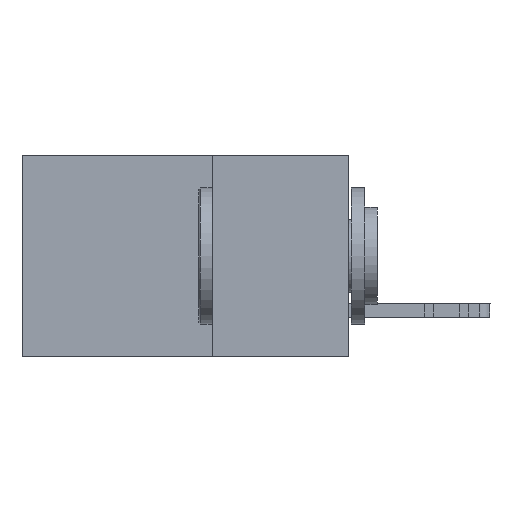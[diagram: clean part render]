
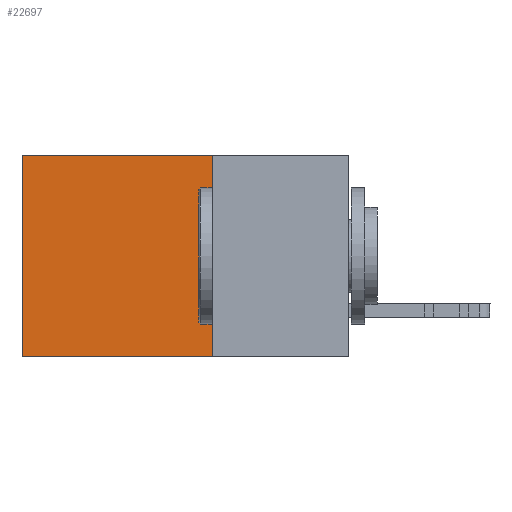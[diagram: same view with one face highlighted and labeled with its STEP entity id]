
A CAD part, left-side view. The second image highlights one B-rep face of the part: STEP entity #22697.
In plain terms, the highlighted planar face has unit normal (-1, 0, 0).
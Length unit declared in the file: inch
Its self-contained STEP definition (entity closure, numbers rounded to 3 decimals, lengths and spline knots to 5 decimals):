
#252 = VERTEX_POINT ( 'NONE', #21242 ) ;
#1880 = ORIENTED_EDGE ( 'NONE', *, *, #21041, .F. ) ;
#3267 = CARTESIAN_POINT ( 'NONE',  ( 0.2615, 0.25, -0.37 ) ) ;
#6181 = LINE ( 'NONE', #14293, #18385 ) ;
#7783 = VERTEX_POINT ( 'NONE', #18566 ) ;
#7862 = DIRECTION ( 'NONE',  ( 0., 0., -1. ) ) ;
#8875 = VERTEX_POINT ( 'NONE', #10356 ) ;
#9104 = AXIS2_PLACEMENT_3D ( 'NONE', #13878, #12019, #26201 ) ;
#9757 = FACE_OUTER_BOUND ( 'NONE', #20924, .T. ) ;
#10244 = ORIENTED_EDGE ( 'NONE', *, *, #13152, .T. ) ;
#10356 = CARTESIAN_POINT ( 'NONE',  ( 0.2615, 0.6, -0.37 ) ) ;
#11650 = DIRECTION ( 'NONE',  ( 0., 1., 0. ) ) ;
#12019 = DIRECTION ( 'NONE',  ( 1., 0., 0. ) ) ;
#12041 = VECTOR ( 'NONE', #7862, 39.37008 ) ;
#12356 = CARTESIAN_POINT ( 'NONE',  ( 0.2615, 0.25, -0.37 ) ) ;
#12427 = VECTOR ( 'NONE', #11650, 39.37008 ) ;
#13152 = EDGE_CURVE ( 'NONE', #7783, #8875, #13577, .T. ) ;
#13577 = LINE ( 'NONE', #25514, #12041 ) ;
#13782 = DIRECTION ( 'NONE',  ( 0., 1., 0. ) ) ;
#13878 = CARTESIAN_POINT ( 'NONE',  ( 0.2615, 0.25, -0.37 ) ) ;
#14007 = PLANE ( 'NONE',  #9104 ) ;
#14293 = CARTESIAN_POINT ( 'NONE',  ( 0.2615, 0.25, -0.37 ) ) ;
#15036 = ORIENTED_EDGE ( 'NONE', *, *, #20762, .F. ) ;
#15376 = LINE ( 'NONE', #3267, #12427 ) ;
#15894 = DIRECTION ( 'NONE',  ( 0., 0., -1. ) ) ;
#17146 = EDGE_CURVE ( 'NONE', #252, #7783, #17765, .T. ) ;
#17765 = LINE ( 'NONE', #25331, #22706 ) ;
#18164 = VERTEX_POINT ( 'NONE', #12356 ) ;
#18385 = VECTOR ( 'NONE', #15894, 39.37008 ) ;
#18566 = CARTESIAN_POINT ( 'NONE',  ( 0.2615, 0.6, 0. ) ) ;
#20762 = EDGE_CURVE ( 'NONE', #18164, #8875, #15376, .T. ) ;
#20924 = EDGE_LOOP ( 'NONE', ( #10244, #15036, #1880, #25718 ) ) ;
#21041 = EDGE_CURVE ( 'NONE', #252, #18164, #6181, .T. ) ;
#21242 = CARTESIAN_POINT ( 'NONE',  ( 0.2615, 0.25, 0. ) ) ;
#22697 = ADVANCED_FACE ( 'NONE', ( #9757 ), #14007, .F. ) ;
#22706 = VECTOR ( 'NONE', #13782, 39.37008 ) ;
#25331 = CARTESIAN_POINT ( 'NONE',  ( 0.2615, 0.25, 0. ) ) ;
#25514 = CARTESIAN_POINT ( 'NONE',  ( 0.2615, 0.6, -0.37 ) ) ;
#25718 = ORIENTED_EDGE ( 'NONE', *, *, #17146, .T. ) ;
#26201 = DIRECTION ( 'NONE',  ( 0., 0., -1. ) ) ;
